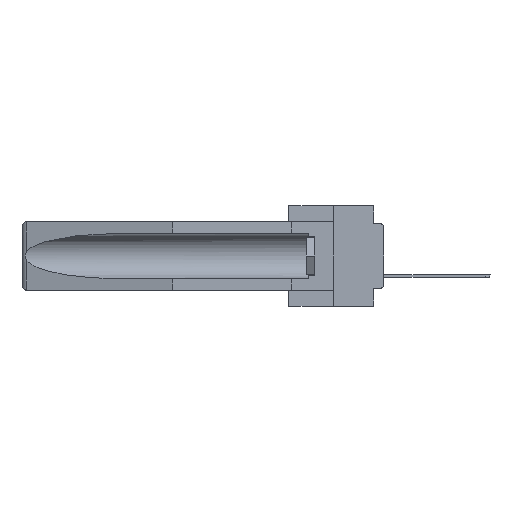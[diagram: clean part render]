
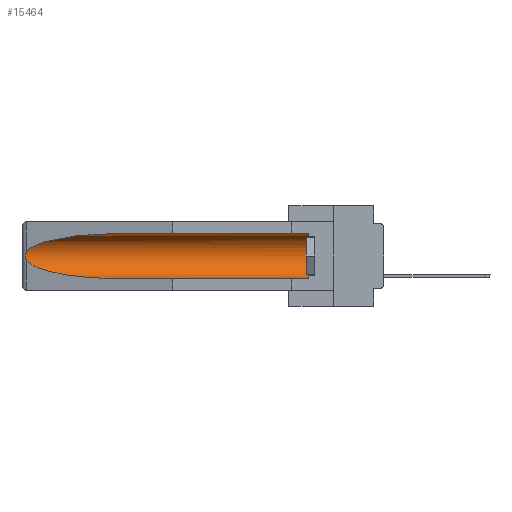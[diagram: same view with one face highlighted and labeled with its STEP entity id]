
A CAD part, left-side view. The second image highlights one B-rep face of the part: STEP entity #15464.
In plain terms, the highlighted cylindrical face has radius 2.857 mm (diameter 5.715 mm), a partial arc.
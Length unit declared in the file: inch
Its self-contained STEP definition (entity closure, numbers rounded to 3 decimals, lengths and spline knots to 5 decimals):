
#74 = DIRECTION ( 'NONE',  ( 0., 1., 0. ) ) ;
#575 = DIRECTION ( 'NONE',  ( 0., 1., 0. ) ) ;
#954 = VERTEX_POINT ( 'NONE', #28353 ) ;
#2068 = ORIENTED_EDGE ( 'NONE', *, *, #28566, .T. ) ;
#3122 = CARTESIAN_POINT ( 'NONE',  ( 0.2675, 1.53308, -0.17534 ) ) ;
#3341 = CARTESIAN_POINT ( 'NONE',  ( 0.155, -0.30754, -0.284 ) ) ;
#3999 = CARTESIAN_POINT ( 'NONE',  ( 0.26537, 1.52718, -0.19328 ) ) ;
#4236 = ORIENTED_EDGE ( 'NONE', *, *, #7665, .T. ) ;
#5111 = FACE_OUTER_BOUND ( 'NONE', #26473, .T. ) ;
#5196 = CARTESIAN_POINT ( 'NONE',  ( 0.26654, 1.53092, -0.15636 ) ) ;
#5285 = VERTEX_POINT ( 'NONE', #10089 ) ;
#5409 = VECTOR ( 'NONE', #8763, 39.37008 ) ;
#5426 = CARTESIAN_POINT ( 'NONE',  ( 0.26537, 1.52718, -0.19328 ) ) ;
#5608 = CARTESIAN_POINT ( 'NONE',  ( 0.2673, 1.53269, -0.17917 ) ) ;
#5891 = VECTOR ( 'NONE', #575, 39.37008 ) ;
#6630 = EDGE_CURVE ( 'NONE', #18685, #20416, #25020, .T. ) ;
#7665 = EDGE_CURVE ( 'NONE', #29091, #5285, #27139, .T. ) ;
#8075 = CARTESIAN_POINT ( 'NONE',  ( 0.26655, 1.53094, -0.18657 ) ) ;
#8081 = LINE ( 'NONE', #28395, #5409 ) ;
#8630 = CARTESIAN_POINT ( 'NONE',  ( 0.155, 0.126, -0.284 ) ) ;
#8763 = DIRECTION ( 'NONE',  ( 0., 1., 0. ) ) ;
#8987 = EDGE_CURVE ( 'NONE', #954, #26716, #23630, .T. ) ;
#9076 = CARTESIAN_POINT ( 'NONE',  ( 0.26537, 1.52718, -0.14972 ) ) ;
#9351 = ORIENTED_EDGE ( 'NONE', *, *, #6630, .T. ) ;
#9779 = CARTESIAN_POINT ( 'NONE',  ( 0.26537, 1.52718, -0.14972 ) ) ;
#10089 = CARTESIAN_POINT ( 'NONE',  ( 0.155, 0.126, -0.059 ) ) ;
#10115 = EDGE_CURVE ( 'NONE', #20416, #954, #15948, .T. ) ;
#10265 = CARTESIAN_POINT ( 'NONE',  ( 0.25451, 1.48313, -0.24835 ) ) ;
#10930 = CARTESIAN_POINT ( 'NONE',  ( 0.21114, 1.30732, -0.059 ) ) ;
#11033 = CARTESIAN_POINT ( 'NONE',  ( 0.155, 1.07973, -0.059 ) ) ;
#12059 = LINE ( 'NONE', #3341, #5891 ) ;
#12988 = CARTESIAN_POINT ( 'NONE',  ( 0.2675, 1.53308, -0.16763 ) ) ;
#13612 = DIRECTION ( 'NONE',  ( 0., 0., 1. ) ) ;
#15464 = ADVANCED_FACE ( 'NONE', ( #5111 ), #23886, .F. ) ;
#15948 = B_SPLINE_CURVE_WITH_KNOTS ( 'NONE', 3,
 ( #9076, #28722, #5196, #25426, #12988, #3122, #5608, #8075, #27816, #3999 ),
 .UNSPECIFIED., .F., .F.,
 ( 4, 2, 2, 2, 4 ),
 ( 0., 0.00029, 0.00058, 0.00087, 0.00117 ),
 .UNSPECIFIED. ) ;
#16589 = ORIENTED_EDGE ( 'NONE', *, *, #10115, .T. ) ;
#18562 = DIRECTION ( 'NONE',  ( 0., -1., 0. ) ) ;
#18685 = VERTEX_POINT ( 'NONE', #27784 ) ;
#19540 = CARTESIAN_POINT ( 'NONE',  ( 0.155, 1.07973, -0.284 ) ) ;
#20194 = CARTESIAN_POINT ( 'NONE',  ( 0.21114, 1.30732, -0.284 ) ) ;
#20289 = CARTESIAN_POINT ( 'NONE',  ( 0.155, 1.07973, -0.284 ) ) ;
#20360 = ORIENTED_EDGE ( 'NONE', *, *, #26231, .F. ) ;
#20416 = VERTEX_POINT ( 'NONE', #9779 ) ;
#20502 = ORIENTED_EDGE ( 'NONE', *, *, #8987, .T. ) ;
#21809 = AXIS2_PLACEMENT_3D ( 'NONE', #28340, #18562, #13612 ) ;
#23215 = CARTESIAN_POINT ( 'NONE',  ( 0.25451, 1.48313, -0.09465 ) ) ;
#23630 =( BOUNDED_CURVE ( )  B_SPLINE_CURVE ( 3, ( #5426, #10265, #20194, #20289 ),
 .UNSPECIFIED., .F., .F. ) 
 B_SPLINE_CURVE_WITH_KNOTS ( ( 4, 4 ),
 ( 0.1948, 1.5708 ),
 .UNSPECIFIED. ) 
 CURVE ( )  GEOMETRIC_REPRESENTATION_ITEM ( )  RATIONAL_B_SPLINE_CURVE ( ( 1., 0.848, 0.848, 1. ) ) 
 REPRESENTATION_ITEM ( '' )  );
#23637 = CARTESIAN_POINT ( 'NONE',  ( 0.155, -0.30754, -0.1715 ) ) ;
#23886 = CYLINDRICAL_SURFACE ( 'NONE', #30117, 0.1125 ) ;
#25020 =( BOUNDED_CURVE ( )  B_SPLINE_CURVE ( 3, ( #11033, #10930, #23215, #25817 ),
 .UNSPECIFIED., .F., .F. ) 
 B_SPLINE_CURVE_WITH_KNOTS ( ( 4, 4 ),
 ( 4.71239, 6.08839 ),
 .UNSPECIFIED. ) 
 CURVE ( )  GEOMETRIC_REPRESENTATION_ITEM ( )  RATIONAL_B_SPLINE_CURVE ( ( 1., 0.848, 0.848, 1. ) ) 
 REPRESENTATION_ITEM ( '' )  );
#25426 = CARTESIAN_POINT ( 'NONE',  ( 0.2673, 1.5327, -0.16383 ) ) ;
#25817 = CARTESIAN_POINT ( 'NONE',  ( 0.26537, 1.52718, -0.14972 ) ) ;
#26231 = EDGE_CURVE ( 'NONE', #29091, #26716, #12059, .T. ) ;
#26473 = EDGE_LOOP ( 'NONE', ( #9351, #16589, #20502, #20360, #4236, #2068 ) ) ;
#26716 = VERTEX_POINT ( 'NONE', #19540 ) ;
#27139 = CIRCLE ( 'NONE', #21809, 0.1125 ) ;
#27784 = CARTESIAN_POINT ( 'NONE',  ( 0.155, 1.07973, -0.059 ) ) ;
#27816 = CARTESIAN_POINT ( 'NONE',  ( 0.26597, 1.5296, -0.19026 ) ) ;
#27862 = DIRECTION ( 'NONE',  ( 0., 0., 1. ) ) ;
#28340 = CARTESIAN_POINT ( 'NONE',  ( 0.155, 0.126, -0.1715 ) ) ;
#28353 = CARTESIAN_POINT ( 'NONE',  ( 0.26537, 1.52718, -0.19328 ) ) ;
#28395 = CARTESIAN_POINT ( 'NONE',  ( 0.155, -0.30754, -0.059 ) ) ;
#28566 = EDGE_CURVE ( 'NONE', #5285, #18685, #8081, .T. ) ;
#28722 = CARTESIAN_POINT ( 'NONE',  ( 0.26597, 1.52961, -0.15275 ) ) ;
#29091 = VERTEX_POINT ( 'NONE', #8630 ) ;
#30117 = AXIS2_PLACEMENT_3D ( 'NONE', #23637, #74, #27862 ) ;
